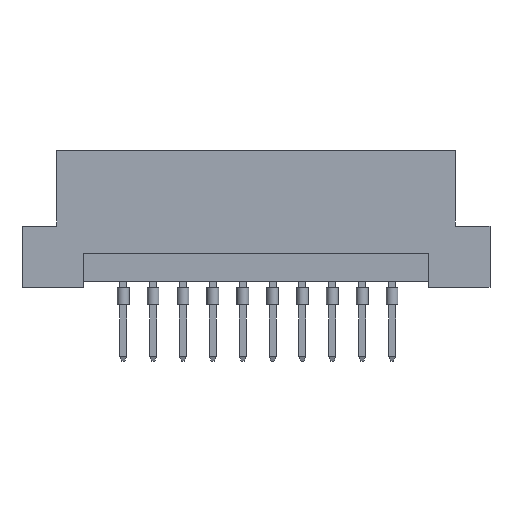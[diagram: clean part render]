
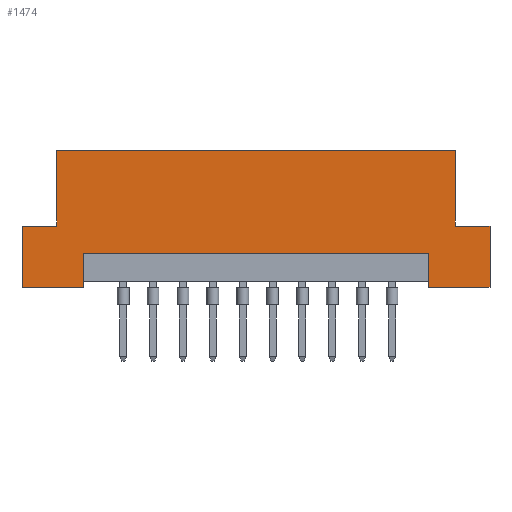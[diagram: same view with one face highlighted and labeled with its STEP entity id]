
A CAD part, front view. The second image highlights one B-rep face of the part: STEP entity #1474.
In plain terms, the highlighted planar face has unit normal (0, -1, 0).
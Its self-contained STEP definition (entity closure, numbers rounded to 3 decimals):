
#2 = CARTESIAN_POINT ( 'NONE',  ( -14.69, 0., 0.5 ) ) ;
#5 = EDGE_CURVE ( 'NONE', #5481, #3496, #2773, .T. ) ;
#148 = EDGE_CURVE ( 'NONE', #2961, #5543, #2311, .T. ) ;
#169 = ORIENTED_EDGE ( 'NONE', *, *, #2280, .F. ) ;
#176 = VECTOR ( 'NONE', #7406, 1000. ) ;
#223 = LINE ( 'NONE', #3230, #2668 ) ;
#256 = EDGE_CURVE ( 'NONE', #3496, #1919, #7202, .T. ) ;
#368 = LINE ( 'NONE', #1504, #7145 ) ;
#411 = CARTESIAN_POINT ( 'NONE',  ( 19.9, 0., 0. ) ) ;
#492 = CARTESIAN_POINT ( 'NONE',  ( -14.69, 0., 2.9 ) ) ;
#528 = VECTOR ( 'NONE', #3089, 1000. ) ;
#635 = CARTESIAN_POINT ( 'NONE',  ( -19.9, 0., 5.2 ) ) ;
#698 = EDGE_CURVE ( 'NONE', #6031, #6685, #2104, .T. ) ;
#707 = CARTESIAN_POINT ( 'NONE',  ( -16.94, 0., 5.2 ) ) ;
#715 = EDGE_CURVE ( 'NONE', #3381, #1149, #5458, .T. ) ;
#1053 = DIRECTION ( 'NONE',  ( 0., 0., 1. ) ) ;
#1149 = VERTEX_POINT ( 'NONE', #5329 ) ;
#1212 = CARTESIAN_POINT ( 'NONE',  ( 14.69, 0., 0.5 ) ) ;
#1370 = VERTEX_POINT ( 'NONE', #7014 ) ;
#1445 = VECTOR ( 'NONE', #7443, 1000. ) ;
#1474 = ADVANCED_FACE ( 'NONE', ( #5131 ), #1580, .F. ) ;
#1504 = CARTESIAN_POINT ( 'NONE',  ( 14.69, 0., 2.9 ) ) ;
#1555 = DIRECTION ( 'NONE',  ( -1., 0., 0. ) ) ;
#1580 = PLANE ( 'NONE',  #1888 ) ;
#1608 = EDGE_CURVE ( 'NONE', #4290, #6031, #6427, .T. ) ;
#1664 = EDGE_CURVE ( 'NONE', #3081, #1370, #3093, .T. ) ;
#1764 = ORIENTED_EDGE ( 'NONE', *, *, #3608, .T. ) ;
#1856 = VECTOR ( 'NONE', #2433, 1000. ) ;
#1888 = AXIS2_PLACEMENT_3D ( 'NONE', #6311, #5810, #1053 ) ;
#1911 = ORIENTED_EDGE ( 'NONE', *, *, #148, .T. ) ;
#1919 = VERTEX_POINT ( 'NONE', #411 ) ;
#2104 = LINE ( 'NONE', #5584, #5917 ) ;
#2140 = CARTESIAN_POINT ( 'NONE',  ( -19.9, 0., 5.2 ) ) ;
#2240 = DIRECTION ( 'NONE',  ( 1., 0., 0. ) ) ;
#2246 = ORIENTED_EDGE ( 'NONE', *, *, #5655, .F. ) ;
#2280 = EDGE_CURVE ( 'NONE', #1919, #5543, #6801, .T. ) ;
#2311 = LINE ( 'NONE', #1212, #1856 ) ;
#2425 = ORIENTED_EDGE ( 'NONE', *, *, #1664, .F. ) ;
#2433 = DIRECTION ( 'NONE',  ( 0., 0., -1. ) ) ;
#2481 = VECTOR ( 'NONE', #3111, 1000. ) ;
#2668 = VECTOR ( 'NONE', #4347, 1000. ) ;
#2686 = DIRECTION ( 'NONE',  ( -1., 0., 0. ) ) ;
#2773 = LINE ( 'NONE', #5130, #3200 ) ;
#2961 = VERTEX_POINT ( 'NONE', #5179 ) ;
#3081 = VERTEX_POINT ( 'NONE', #3857 ) ;
#3089 = DIRECTION ( 'NONE',  ( 0., 0., -1. ) ) ;
#3093 = LINE ( 'NONE', #5969, #3598 ) ;
#3111 = DIRECTION ( 'NONE',  ( 0., 0., 1. ) ) ;
#3200 = VECTOR ( 'NONE', #2240, 1000. ) ;
#3230 = CARTESIAN_POINT ( 'NONE',  ( 16.94, 0., 5.2 ) ) ;
#3237 = CARTESIAN_POINT ( 'NONE',  ( 19.9, 0., 0. ) ) ;
#3364 = EDGE_LOOP ( 'NONE', ( #7435, #1911, #169, #5454, #5126, #1764, #2425, #7164, #5889, #2246, #4097, #4921 ) ) ;
#3381 = VERTEX_POINT ( 'NONE', #635 ) ;
#3435 = LINE ( 'NONE', #5142, #1445 ) ;
#3496 = VERTEX_POINT ( 'NONE', #4854 ) ;
#3598 = VECTOR ( 'NONE', #6553, 1000. ) ;
#3608 = EDGE_CURVE ( 'NONE', #5481, #1370, #223, .T. ) ;
#3616 = LINE ( 'NONE', #707, #2481 ) ;
#3684 = CARTESIAN_POINT ( 'NONE',  ( 14.69, 0., 0. ) ) ;
#3857 = CARTESIAN_POINT ( 'NONE',  ( -16.94, 0., 11.6 ) ) ;
#4097 = ORIENTED_EDGE ( 'NONE', *, *, #698, .F. ) ;
#4186 = CARTESIAN_POINT ( 'NONE',  ( -19.9, 0., 0. ) ) ;
#4290 = VERTEX_POINT ( 'NONE', #492 ) ;
#4347 = DIRECTION ( 'NONE',  ( 0., 0., 1. ) ) ;
#4361 = CARTESIAN_POINT ( 'NONE',  ( -14.69, 0., 0. ) ) ;
#4505 = CARTESIAN_POINT ( 'NONE',  ( -19.9, 0., 0. ) ) ;
#4854 = CARTESIAN_POINT ( 'NONE',  ( 19.9, 0., 5.2 ) ) ;
#4921 = ORIENTED_EDGE ( 'NONE', *, *, #1608, .F. ) ;
#5126 = ORIENTED_EDGE ( 'NONE', *, *, #5, .F. ) ;
#5130 = CARTESIAN_POINT ( 'NONE',  ( 19.9, 0., 5.2 ) ) ;
#5131 = FACE_OUTER_BOUND ( 'NONE', #3364, .T. ) ;
#5142 = CARTESIAN_POINT ( 'NONE',  ( -19.9, 0., 0. ) ) ;
#5179 = CARTESIAN_POINT ( 'NONE',  ( 14.69, 0., 2.9 ) ) ;
#5276 = DIRECTION ( 'NONE',  ( 0., 0., -1. ) ) ;
#5329 = CARTESIAN_POINT ( 'NONE',  ( -16.94, 0., 5.2 ) ) ;
#5454 = ORIENTED_EDGE ( 'NONE', *, *, #256, .F. ) ;
#5458 = LINE ( 'NONE', #2140, #176 ) ;
#5481 = VERTEX_POINT ( 'NONE', #7297 ) ;
#5543 = VERTEX_POINT ( 'NONE', #3684 ) ;
#5584 = CARTESIAN_POINT ( 'NONE',  ( -19.9, 0., 0. ) ) ;
#5655 = EDGE_CURVE ( 'NONE', #6685, #3381, #3435, .T. ) ;
#5810 = DIRECTION ( 'NONE',  ( 0., 1., 0. ) ) ;
#5889 = ORIENTED_EDGE ( 'NONE', *, *, #715, .F. ) ;
#5917 = VECTOR ( 'NONE', #1555, 1000. ) ;
#5930 = VECTOR ( 'NONE', #5276, 1000. ) ;
#5969 = CARTESIAN_POINT ( 'NONE',  ( -19.9, 0., 11.6 ) ) ;
#6031 = VERTEX_POINT ( 'NONE', #4361 ) ;
#6154 = VECTOR ( 'NONE', #6760, 1000. ) ;
#6311 = CARTESIAN_POINT ( 'NONE',  ( -19.9, 0., 11.6 ) ) ;
#6427 = LINE ( 'NONE', #2, #5930 ) ;
#6457 = EDGE_CURVE ( 'NONE', #2961, #4290, #368, .T. ) ;
#6553 = DIRECTION ( 'NONE',  ( 1., 0., 0. ) ) ;
#6660 = EDGE_CURVE ( 'NONE', #1149, #3081, #3616, .T. ) ;
#6685 = VERTEX_POINT ( 'NONE', #4186 ) ;
#6760 = DIRECTION ( 'NONE',  ( -1., 0., 0. ) ) ;
#6801 = LINE ( 'NONE', #4505, #6154 ) ;
#7014 = CARTESIAN_POINT ( 'NONE',  ( 16.94, 0., 11.6 ) ) ;
#7145 = VECTOR ( 'NONE', #2686, 1000. ) ;
#7164 = ORIENTED_EDGE ( 'NONE', *, *, #6660, .F. ) ;
#7202 = LINE ( 'NONE', #3237, #528 ) ;
#7297 = CARTESIAN_POINT ( 'NONE',  ( 16.94, 0., 5.2 ) ) ;
#7406 = DIRECTION ( 'NONE',  ( 1., 0., 0. ) ) ;
#7435 = ORIENTED_EDGE ( 'NONE', *, *, #6457, .F. ) ;
#7443 = DIRECTION ( 'NONE',  ( 0., 0., 1. ) ) ;
